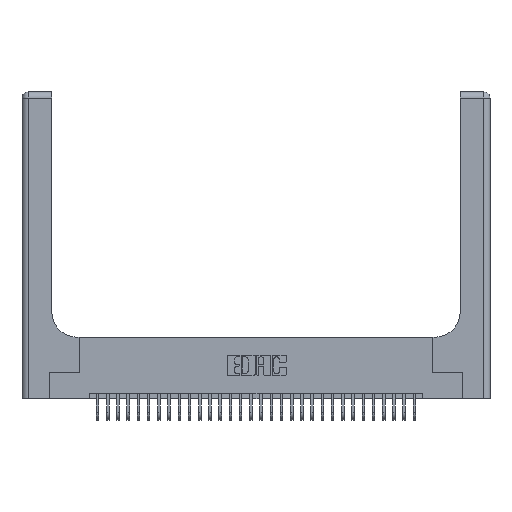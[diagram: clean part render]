
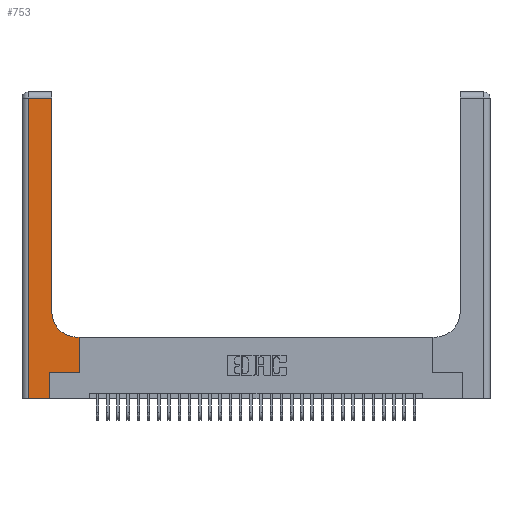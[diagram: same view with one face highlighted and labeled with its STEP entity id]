
A CAD part, top view. The second image highlights one B-rep face of the part: STEP entity #753.
In plain terms, the highlighted planar face has unit normal (0, 0, 1).
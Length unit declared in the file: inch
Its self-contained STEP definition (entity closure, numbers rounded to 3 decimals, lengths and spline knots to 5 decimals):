
#753 = ADVANCED_FACE ( 'NONE', ( #30177 ), #5859, .F. ) ;
#2479 = DIRECTION ( 'NONE',  ( -1., 0., 0. ) ) ;
#2956 = VERTEX_POINT ( 'NONE', #26233 ) ;
#3053 = DIRECTION ( 'NONE',  ( 1., 0., 0. ) ) ;
#3172 = CARTESIAN_POINT ( 'NONE',  ( 0., 3., 0.37 ) ) ;
#3276 = CARTESIAN_POINT ( 'NONE',  ( 0.269, 0.25, 0.37 ) ) ;
#3291 = VECTOR ( 'NONE', #29193, 39.37008 ) ;
#3551 = EDGE_LOOP ( 'NONE', ( #31622, #31463, #16236, #16657, #26200, #27187, #11775, #31653, #11799 ) ) ;
#4259 = AXIS2_PLACEMENT_3D ( 'NONE', #3172, #8746, #16416 ) ;
#5787 = EDGE_CURVE ( 'NONE', #29804, #2956, #12818, .T. ) ;
#5853 = LINE ( 'NONE', #6334, #21995 ) ;
#5859 = PLANE ( 'NONE',  #4259 ) ;
#6261 = EDGE_CURVE ( 'NONE', #26207, #16248, #21990, .T. ) ;
#6334 = CARTESIAN_POINT ( 'NONE',  ( 0.269, 0., 0.37 ) ) ;
#6342 = VERTEX_POINT ( 'NONE', #7050 ) ;
#6633 = CARTESIAN_POINT ( 'NONE',  ( 0.5585, 0.6, 0.37 ) ) ;
#7050 = CARTESIAN_POINT ( 'NONE',  ( 0.269, 0., 0.37 ) ) ;
#7247 = DIRECTION ( 'NONE',  ( -1., 0., 0. ) ) ;
#7531 = VECTOR ( 'NONE', #16256, 39.37008 ) ;
#7558 = DIRECTION ( 'NONE',  ( 1., 0., 0. ) ) ;
#7639 = CARTESIAN_POINT ( 'NONE',  ( 0.06, 2.94, 0.37 ) ) ;
#8171 = VECTOR ( 'NONE', #3053, 39.37008 ) ;
#8330 = EDGE_CURVE ( 'NONE', #2956, #6342, #16666, .T. ) ;
#8617 = CARTESIAN_POINT ( 'NONE',  ( 0., 0., 0.37 ) ) ;
#8746 = DIRECTION ( 'NONE',  ( 0., 0., -1. ) ) ;
#8928 = CARTESIAN_POINT ( 'NONE',  ( 0.2915, 2.94, 0.37 ) ) ;
#8947 = EDGE_CURVE ( 'NONE', #11691, #13021, #10048, .T. ) ;
#10048 = LINE ( 'NONE', #23481, #29685 ) ;
#10240 = VECTOR ( 'NONE', #29145, 39.37008 ) ;
#11691 = VERTEX_POINT ( 'NONE', #6633 ) ;
#11775 = ORIENTED_EDGE ( 'NONE', *, *, #28911, .T. ) ;
#11799 = ORIENTED_EDGE ( 'NONE', *, *, #14972, .T. ) ;
#12818 = LINE ( 'NONE', #22402, #15625 ) ;
#13021 = VERTEX_POINT ( 'NONE', #15303 ) ;
#13380 = VECTOR ( 'NONE', #2479, 39.37008 ) ;
#13654 = CARTESIAN_POINT ( 'NONE',  ( 0.2915, 3., 0.37 ) ) ;
#14191 = LINE ( 'NONE', #28562, #13380 ) ;
#14277 = DIRECTION ( 'NONE',  ( 0., 1., 0. ) ) ;
#14972 = EDGE_CURVE ( 'NONE', #13021, #26207, #16991, .T. ) ;
#15303 = CARTESIAN_POINT ( 'NONE',  ( 0.5415, 0.6, 0.37 ) ) ;
#15625 = VECTOR ( 'NONE', #17075, 39.37008 ) ;
#16236 = ORIENTED_EDGE ( 'NONE', *, *, #5787, .T. ) ;
#16248 = VERTEX_POINT ( 'NONE', #8928 ) ;
#16256 = DIRECTION ( 'NONE',  ( 0., 1., 0. ) ) ;
#16416 = DIRECTION ( 'NONE',  ( -1., 0., 0. ) ) ;
#16657 = ORIENTED_EDGE ( 'NONE', *, *, #8330, .T. ) ;
#16666 = LINE ( 'NONE', #8617, #10240 ) ;
#16991 = CIRCLE ( 'NONE', #20069, 0.25 ) ;
#17075 = DIRECTION ( 'NONE',  ( 0., -1., 0. ) ) ;
#19466 = LINE ( 'NONE', #3276, #8171 ) ;
#20069 = AXIS2_PLACEMENT_3D ( 'NONE', #22942, #23163, #7558 ) ;
#20953 = EDGE_CURVE ( 'NONE', #6342, #25639, #5853, .T. ) ;
#21064 = LINE ( 'NONE', #29296, #3291 ) ;
#21532 = CARTESIAN_POINT ( 'NONE',  ( 0.2915, 0.85, 0.37 ) ) ;
#21990 = LINE ( 'NONE', #13654, #7531 ) ;
#21995 = VECTOR ( 'NONE', #14277, 39.37008 ) ;
#22402 = CARTESIAN_POINT ( 'NONE',  ( 0.06, 3., 0.37 ) ) ;
#22942 = CARTESIAN_POINT ( 'NONE',  ( 0.5415, 0.85, 0.37 ) ) ;
#23163 = DIRECTION ( 'NONE',  ( 0., 0., -1. ) ) ;
#23481 = CARTESIAN_POINT ( 'NONE',  ( 0.2915, 0.6, 0.37 ) ) ;
#24365 = EDGE_CURVE ( 'NONE', #25639, #30957, #19466, .T. ) ;
#24884 = EDGE_CURVE ( 'NONE', #16248, #29804, #14191, .T. ) ;
#25639 = VERTEX_POINT ( 'NONE', #29748 ) ;
#26200 = ORIENTED_EDGE ( 'NONE', *, *, #20953, .T. ) ;
#26207 = VERTEX_POINT ( 'NONE', #21532 ) ;
#26233 = CARTESIAN_POINT ( 'NONE',  ( 0.06, 0., 0.37 ) ) ;
#27187 = ORIENTED_EDGE ( 'NONE', *, *, #24365, .T. ) ;
#28005 = CARTESIAN_POINT ( 'NONE',  ( 0.5585, 0.25, 0.37 ) ) ;
#28562 = CARTESIAN_POINT ( 'NONE',  ( 0., 2.94, 0.37 ) ) ;
#28911 = EDGE_CURVE ( 'NONE', #30957, #11691, #21064, .T. ) ;
#29145 = DIRECTION ( 'NONE',  ( 1., 0., 0. ) ) ;
#29193 = DIRECTION ( 'NONE',  ( 0., 1., 0. ) ) ;
#29296 = CARTESIAN_POINT ( 'NONE',  ( 0.5585, 0.25, 0.37 ) ) ;
#29685 = VECTOR ( 'NONE', #7247, 39.37008 ) ;
#29748 = CARTESIAN_POINT ( 'NONE',  ( 0.269, 0.25, 0.37 ) ) ;
#29804 = VERTEX_POINT ( 'NONE', #7639 ) ;
#30177 = FACE_OUTER_BOUND ( 'NONE', #3551, .T. ) ;
#30957 = VERTEX_POINT ( 'NONE', #28005 ) ;
#31463 = ORIENTED_EDGE ( 'NONE', *, *, #24884, .T. ) ;
#31622 = ORIENTED_EDGE ( 'NONE', *, *, #6261, .T. ) ;
#31653 = ORIENTED_EDGE ( 'NONE', *, *, #8947, .T. ) ;
